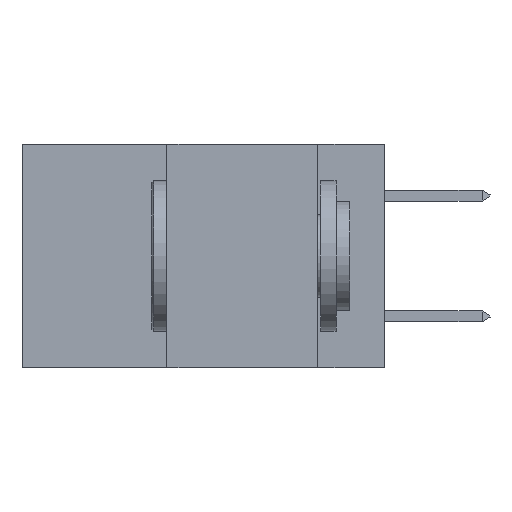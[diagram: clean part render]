
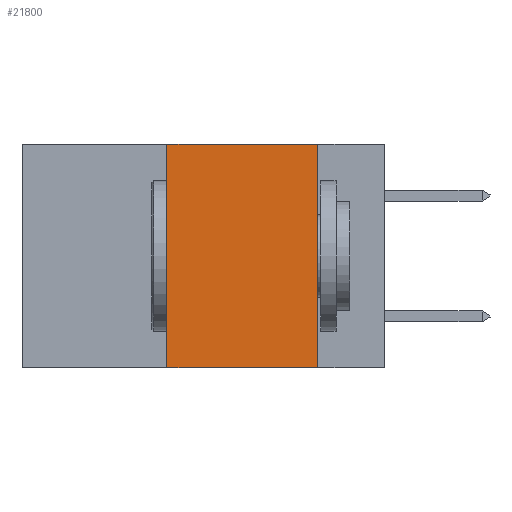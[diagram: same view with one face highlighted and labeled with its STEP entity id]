
A CAD part, left-side view. The second image highlights one B-rep face of the part: STEP entity #21800.
In plain terms, the highlighted planar face has unit normal (-1, 0, 0).
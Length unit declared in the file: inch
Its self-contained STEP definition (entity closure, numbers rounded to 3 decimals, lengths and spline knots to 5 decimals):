
#50 = DIRECTION ( 'NONE',  ( 0., -1., 0. ) ) ;
#1776 = DIRECTION ( 'NONE',  ( 0., -1., 0. ) ) ;
#3125 = VECTOR ( 'NONE', #12398, 39.37008 ) ;
#3167 = ORIENTED_EDGE ( 'NONE', *, *, #3238, .F. ) ;
#3238 = EDGE_CURVE ( 'NONE', #8058, #13113, #22821, .T. ) ;
#3754 = ORIENTED_EDGE ( 'NONE', *, *, #22690, .F. ) ;
#4351 = ORIENTED_EDGE ( 'NONE', *, *, #23923, .T. ) ;
#4465 = VECTOR ( 'NONE', #50, 39.37008 ) ;
#5265 = EDGE_CURVE ( 'NONE', #17844, #8058, #19824, .T. ) ;
#5967 = CARTESIAN_POINT ( 'NONE',  ( 0., 0.6, 0. ) ) ;
#6255 = CARTESIAN_POINT ( 'NONE',  ( 0., 0.11, -0.37 ) ) ;
#6774 = AXIS2_PLACEMENT_3D ( 'NONE', #5967, #18931, #7813 ) ;
#7393 = CARTESIAN_POINT ( 'NONE',  ( 0., 0.6, -0.37 ) ) ;
#7813 = DIRECTION ( 'NONE',  ( 0., 0., -1. ) ) ;
#8017 = VECTOR ( 'NONE', #1776, 39.37008 ) ;
#8048 = VECTOR ( 'NONE', #8345, 39.37008 ) ;
#8058 = VERTEX_POINT ( 'NONE', #20519 ) ;
#8089 = LINE ( 'NONE', #9344, #3125 ) ;
#8345 = DIRECTION ( 'NONE',  ( 0., 0., -1. ) ) ;
#8604 = LINE ( 'NONE', #7393, #8017 ) ;
#8716 = CARTESIAN_POINT ( 'NONE',  ( 0., 0.11, 0. ) ) ;
#9344 = CARTESIAN_POINT ( 'NONE',  ( 0., 0.36, 0. ) ) ;
#9420 = CARTESIAN_POINT ( 'NONE',  ( 0., 0.6, 0. ) ) ;
#11402 = PLANE ( 'NONE',  #6774 ) ;
#12162 = VERTEX_POINT ( 'NONE', #13118 ) ;
#12398 = DIRECTION ( 'NONE',  ( 0., 0., 1. ) ) ;
#13113 = VERTEX_POINT ( 'NONE', #6255 ) ;
#13118 = CARTESIAN_POINT ( 'NONE',  ( 0., 0.36, -0.37 ) ) ;
#16693 = CARTESIAN_POINT ( 'NONE',  ( 0., 0.36, 0. ) ) ;
#17368 = EDGE_LOOP ( 'NONE', ( #3167, #22911, #3754, #4351 ) ) ;
#17844 = VERTEX_POINT ( 'NONE', #16693 ) ;
#18931 = DIRECTION ( 'NONE',  ( 1., 0., 0. ) ) ;
#19824 = LINE ( 'NONE', #9420, #4465 ) ;
#20519 = CARTESIAN_POINT ( 'NONE',  ( 0., 0.11, 0. ) ) ;
#21800 = ADVANCED_FACE ( 'NONE', ( #24041 ), #11402, .F. ) ;
#22690 = EDGE_CURVE ( 'NONE', #12162, #17844, #8089, .T. ) ;
#22821 = LINE ( 'NONE', #8716, #8048 ) ;
#22911 = ORIENTED_EDGE ( 'NONE', *, *, #5265, .F. ) ;
#23923 = EDGE_CURVE ( 'NONE', #12162, #13113, #8604, .T. ) ;
#24041 = FACE_OUTER_BOUND ( 'NONE', #17368, .T. ) ;
